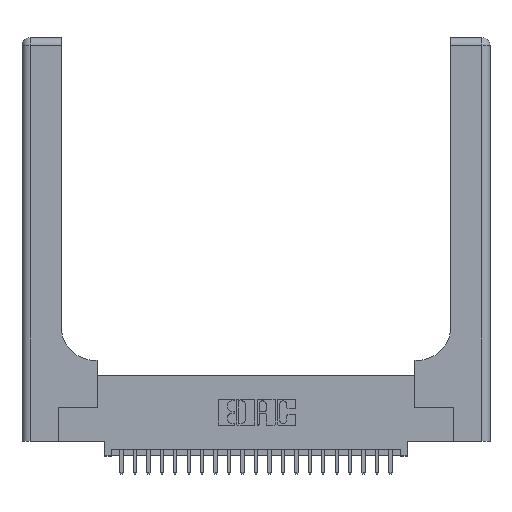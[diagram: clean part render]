
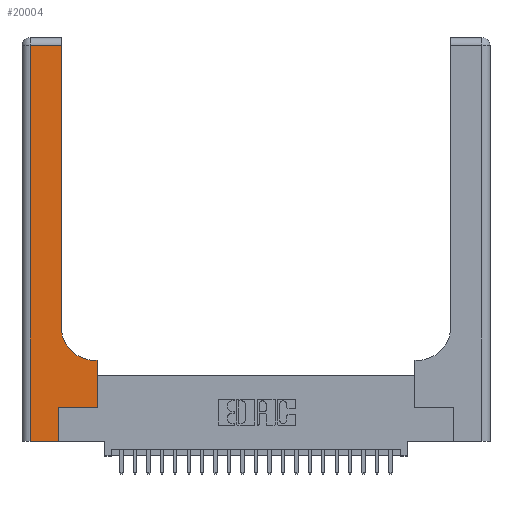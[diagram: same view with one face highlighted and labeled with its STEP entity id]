
A CAD part, top view. The second image highlights one B-rep face of the part: STEP entity #20004.
In plain terms, the highlighted planar face has unit normal (0, 0, 1).
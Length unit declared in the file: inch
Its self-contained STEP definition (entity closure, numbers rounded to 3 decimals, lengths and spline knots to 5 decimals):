
#189 = EDGE_CURVE ( 'NONE', #19358, #23624, #23903, .T. ) ;
#634 = EDGE_CURVE ( 'NONE', #10719, #19358, #920, .T. ) ;
#920 = LINE ( 'NONE', #4569, #21138 ) ;
#1056 = CARTESIAN_POINT ( 'NONE',  ( 0.5415, 0.85, 0.37 ) ) ;
#1413 = VERTEX_POINT ( 'NONE', #12732 ) ;
#3725 = ORIENTED_EDGE ( 'NONE', *, *, #16930, .T. ) ;
#4123 = VECTOR ( 'NONE', #16863, 39.37008 ) ;
#4138 = EDGE_CURVE ( 'NONE', #10961, #1413, #20465, .T. ) ;
#4344 = AXIS2_PLACEMENT_3D ( 'NONE', #18183, #14412, #6767 ) ;
#4569 = CARTESIAN_POINT ( 'NONE',  ( 0.269, 0.25, 0.37 ) ) ;
#4766 = ORIENTED_EDGE ( 'NONE', *, *, #15128, .T. ) ;
#5314 = CARTESIAN_POINT ( 'NONE',  ( 0.5585, 0.6, 0.37 ) ) ;
#5897 = CARTESIAN_POINT ( 'NONE',  ( 0.06, 3., 0.37 ) ) ;
#6264 = ORIENTED_EDGE ( 'NONE', *, *, #23276, .T. ) ;
#6356 = DIRECTION ( 'NONE',  ( 0., 1., 0. ) ) ;
#6439 = EDGE_LOOP ( 'NONE', ( #16506, #21066, #6264, #3725, #11735, #17814, #13449, #4766, #16585 ) ) ;
#6767 = DIRECTION ( 'NONE',  ( -1., 0., 0. ) ) ;
#6910 = VECTOR ( 'NONE', #7530, 39.37008 ) ;
#7376 = VECTOR ( 'NONE', #21126, 39.37008 ) ;
#7478 = CARTESIAN_POINT ( 'NONE',  ( 0.2915, 0.85, 0.37 ) ) ;
#7500 = VECTOR ( 'NONE', #7868, 39.37008 ) ;
#7530 = DIRECTION ( 'NONE',  ( -1., 0., 0. ) ) ;
#7868 = DIRECTION ( 'NONE',  ( 0., 1., 0. ) ) ;
#8221 = EDGE_CURVE ( 'NONE', #16582, #10961, #21489, .T. ) ;
#8382 = CARTESIAN_POINT ( 'NONE',  ( 0.06, 0., 0.37 ) ) ;
#8432 = PLANE ( 'NONE',  #4344 ) ;
#9093 = CARTESIAN_POINT ( 'NONE',  ( 0., 0., 0.37 ) ) ;
#9269 = CARTESIAN_POINT ( 'NONE',  ( 0.269, 0.25, 0.37 ) ) ;
#9518 = CARTESIAN_POINT ( 'NONE',  ( 0.2915, 0.6, 0.37 ) ) ;
#9996 = VECTOR ( 'NONE', #16725, 39.37008 ) ;
#10365 = DIRECTION ( 'NONE',  ( 0., 0., -1. ) ) ;
#10719 = VERTEX_POINT ( 'NONE', #9269 ) ;
#10901 = CARTESIAN_POINT ( 'NONE',  ( 0.06, 2.94, 0.37 ) ) ;
#10961 = VERTEX_POINT ( 'NONE', #7478 ) ;
#11110 = CARTESIAN_POINT ( 'NONE',  ( 0.2915, 3., 0.37 ) ) ;
#11530 = FACE_OUTER_BOUND ( 'NONE', #6439, .T. ) ;
#11551 = LINE ( 'NONE', #9093, #4123 ) ;
#11664 = LINE ( 'NONE', #5897, #16470 ) ;
#11735 = ORIENTED_EDGE ( 'NONE', *, *, #20326, .T. ) ;
#11820 = LINE ( 'NONE', #13703, #7376 ) ;
#12536 = EDGE_CURVE ( 'NONE', #1413, #24589, #14466, .T. ) ;
#12732 = CARTESIAN_POINT ( 'NONE',  ( 0.2915, 2.94, 0.37 ) ) ;
#13449 = ORIENTED_EDGE ( 'NONE', *, *, #189, .T. ) ;
#13703 = CARTESIAN_POINT ( 'NONE',  ( 0.269, 0., 0.37 ) ) ;
#14015 = DIRECTION ( 'NONE',  ( 1., 0., 0. ) ) ;
#14412 = DIRECTION ( 'NONE',  ( 0., 0., -1. ) ) ;
#14466 = LINE ( 'NONE', #24283, #9996 ) ;
#15128 = EDGE_CURVE ( 'NONE', #23624, #16582, #22087, .T. ) ;
#15417 = AXIS2_PLACEMENT_3D ( 'NONE', #1056, #10365, #14015 ) ;
#16059 = CARTESIAN_POINT ( 'NONE',  ( 0.5585, 0.25, 0.37 ) ) ;
#16127 = CARTESIAN_POINT ( 'NONE',  ( 0.5585, 0.25, 0.37 ) ) ;
#16470 = VECTOR ( 'NONE', #23055, 39.37008 ) ;
#16506 = ORIENTED_EDGE ( 'NONE', *, *, #4138, .T. ) ;
#16582 = VERTEX_POINT ( 'NONE', #21511 ) ;
#16585 = ORIENTED_EDGE ( 'NONE', *, *, #8221, .T. ) ;
#16627 = VECTOR ( 'NONE', #6356, 39.37008 ) ;
#16725 = DIRECTION ( 'NONE',  ( -1., 0., 0. ) ) ;
#16863 = DIRECTION ( 'NONE',  ( 1., 0., 0. ) ) ;
#16930 = EDGE_CURVE ( 'NONE', #23333, #24509, #11551, .T. ) ;
#17814 = ORIENTED_EDGE ( 'NONE', *, *, #634, .T. ) ;
#18183 = CARTESIAN_POINT ( 'NONE',  ( 0., 3., 0.37 ) ) ;
#19358 = VERTEX_POINT ( 'NONE', #16127 ) ;
#20004 = ADVANCED_FACE ( 'NONE', ( #11530 ), #8432, .F. ) ;
#20326 = EDGE_CURVE ( 'NONE', #24509, #10719, #11820, .T. ) ;
#20465 = LINE ( 'NONE', #11110, #16627 ) ;
#21066 = ORIENTED_EDGE ( 'NONE', *, *, #12536, .T. ) ;
#21126 = DIRECTION ( 'NONE',  ( 0., 1., 0. ) ) ;
#21138 = VECTOR ( 'NONE', #21546, 39.37008 ) ;
#21312 = CARTESIAN_POINT ( 'NONE',  ( 0.269, 0., 0.37 ) ) ;
#21489 = CIRCLE ( 'NONE', #15417, 0.25 ) ;
#21511 = CARTESIAN_POINT ( 'NONE',  ( 0.5415, 0.6, 0.37 ) ) ;
#21546 = DIRECTION ( 'NONE',  ( 1., 0., 0. ) ) ;
#22087 = LINE ( 'NONE', #9518, #6910 ) ;
#23055 = DIRECTION ( 'NONE',  ( 0., -1., 0. ) ) ;
#23276 = EDGE_CURVE ( 'NONE', #24589, #23333, #11664, .T. ) ;
#23333 = VERTEX_POINT ( 'NONE', #8382 ) ;
#23624 = VERTEX_POINT ( 'NONE', #5314 ) ;
#23903 = LINE ( 'NONE', #16059, #7500 ) ;
#24283 = CARTESIAN_POINT ( 'NONE',  ( 0., 2.94, 0.37 ) ) ;
#24509 = VERTEX_POINT ( 'NONE', #21312 ) ;
#24589 = VERTEX_POINT ( 'NONE', #10901 ) ;
